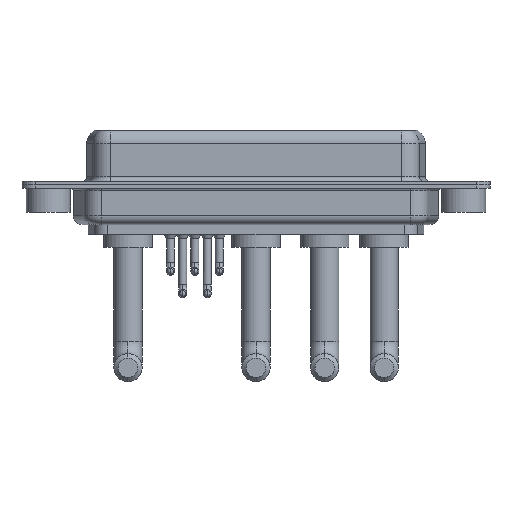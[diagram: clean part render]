
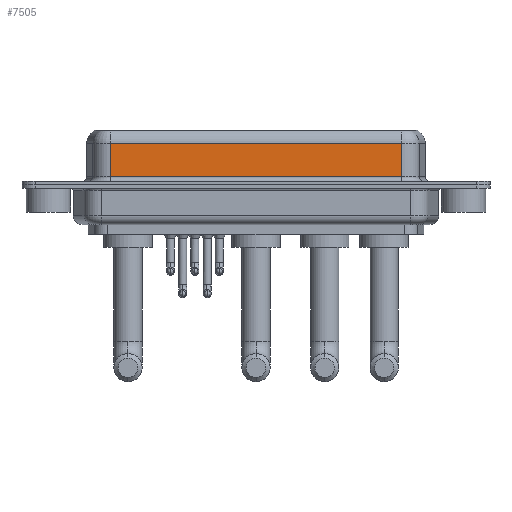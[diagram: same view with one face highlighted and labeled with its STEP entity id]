
A CAD part, front view. The second image highlights one B-rep face of the part: STEP entity #7505.
In plain terms, the highlighted planar face has unit normal (0, -1, 0).
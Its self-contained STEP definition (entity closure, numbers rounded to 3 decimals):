
#298 = VERTEX_POINT ( 'NONE', #12164 ) ;
#432 = DIRECTION ( 'NONE',  ( 0., 0., -1. ) ) ;
#582 = CARTESIAN_POINT ( 'NONE',  ( 40.037, -3.95, 0.9 ) ) ;
#596 = AXIS2_PLACEMENT_3D ( 'NONE', #9757, #8706, #8447 ) ;
#624 = CARTESIAN_POINT ( 'NONE',  ( 40.037, -3.95, 4.65 ) ) ;
#2345 = DIRECTION ( 'NONE',  ( 0., 0., -1. ) ) ;
#2431 = LINE ( 'NONE', #7771, #7221 ) ;
#2516 = EDGE_CURVE ( 'NONE', #14562, #2724, #2431, .T. ) ;
#2724 = VERTEX_POINT ( 'NONE', #582 ) ;
#2782 = EDGE_LOOP ( 'NONE', ( #6702, #12650, #15100, #3909 ) ) ;
#2811 = CARTESIAN_POINT ( 'NONE',  ( 40.037, -3.95, 4.65 ) ) ;
#3909 = ORIENTED_EDGE ( 'NONE', *, *, #8921, .T. ) ;
#5195 = EDGE_CURVE ( 'NONE', #14562, #298, #8843, .T. ) ;
#6702 = ORIENTED_EDGE ( 'NONE', *, *, #2516, .F. ) ;
#7221 = VECTOR ( 'NONE', #2345, 1000. ) ;
#7505 = ADVANCED_FACE ( 'NONE', ( #8541 ), #10016, .F. ) ;
#7531 = CARTESIAN_POINT ( 'NONE',  ( 40.037, -3.95, 0.9 ) ) ;
#7771 = CARTESIAN_POINT ( 'NONE',  ( 40.037, -3.95, 6.4 ) ) ;
#7972 = EDGE_CURVE ( 'NONE', #298, #14514, #14995, .T. ) ;
#8447 = DIRECTION ( 'NONE',  ( 0., 0., 1. ) ) ;
#8541 = FACE_OUTER_BOUND ( 'NONE', #2782, .T. ) ;
#8706 = DIRECTION ( 'NONE',  ( 0., 1., 0. ) ) ;
#8843 = LINE ( 'NONE', #624, #14461 ) ;
#8921 = EDGE_CURVE ( 'NONE', #14514, #2724, #12928, .T. ) ;
#9757 = CARTESIAN_POINT ( 'NONE',  ( 40.037, -3.95, 6.4 ) ) ;
#10016 = PLANE ( 'NONE',  #596 ) ;
#11705 = DIRECTION ( 'NONE',  ( 1., 0., 0. ) ) ;
#12164 = CARTESIAN_POINT ( 'NONE',  ( 7.013, -3.95, 4.65 ) ) ;
#12650 = ORIENTED_EDGE ( 'NONE', *, *, #5195, .T. ) ;
#12928 = LINE ( 'NONE', #7531, #15948 ) ;
#13686 = CARTESIAN_POINT ( 'NONE',  ( 7.013, -3.95, 6.4 ) ) ;
#14255 = VECTOR ( 'NONE', #432, 1000. ) ;
#14461 = VECTOR ( 'NONE', #15095, 1000. ) ;
#14514 = VERTEX_POINT ( 'NONE', #14931 ) ;
#14562 = VERTEX_POINT ( 'NONE', #2811 ) ;
#14931 = CARTESIAN_POINT ( 'NONE',  ( 7.013, -3.95, 0.9 ) ) ;
#14995 = LINE ( 'NONE', #13686, #14255 ) ;
#15095 = DIRECTION ( 'NONE',  ( -1., 0., 0. ) ) ;
#15100 = ORIENTED_EDGE ( 'NONE', *, *, #7972, .T. ) ;
#15948 = VECTOR ( 'NONE', #11705, 1000. ) ;
